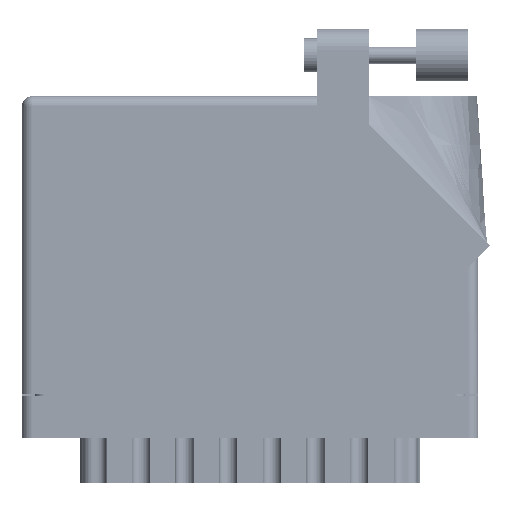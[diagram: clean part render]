
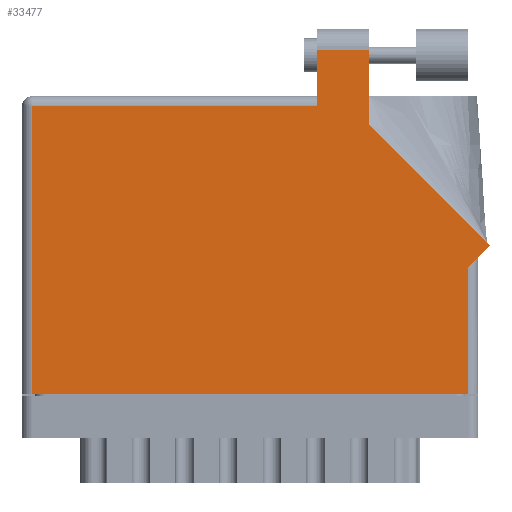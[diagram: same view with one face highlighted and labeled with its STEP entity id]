
A CAD part, front view. The second image highlights one B-rep face of the part: STEP entity #33477.
In plain terms, the highlighted face is planar.
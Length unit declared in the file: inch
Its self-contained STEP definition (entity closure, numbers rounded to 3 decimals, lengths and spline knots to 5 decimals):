
#1306 = DIRECTION ( 'NONE',  ( -1., 0., 0. ) ) ;
#2061 = DIRECTION ( 'NONE',  ( 0., 0., -1. ) ) ;
#2221 = VECTOR ( 'NONE', #69357, 39.37008 ) ;
#2940 = LINE ( 'NONE', #4079, #55872 ) ;
#4079 = CARTESIAN_POINT ( 'NONE',  ( 1.758, 2.05, 0. ) ) ;
#4353 = LINE ( 'NONE', #40347, #47713 ) ;
#5128 = ORIENTED_EDGE ( 'NONE', *, *, #47192, .T. ) ;
#6887 = CARTESIAN_POINT ( 'NONE',  ( 2.78871, 0.88571, 0. ) ) ;
#7478 = CARTESIAN_POINT ( 'NONE',  ( 0., 1.775, 0. ) ) ;
#8023 = DIRECTION ( 'NONE',  ( -0.707, 0.707, 0. ) ) ;
#9760 = CARTESIAN_POINT ( 'NONE',  ( 2.065, 1.60942, 0. ) ) ;
#12883 = EDGE_CURVE ( 'NONE', #18476, #69087, #34886, .T. ) ;
#13720 = LINE ( 'NONE', #59563, #61947 ) ;
#16546 = CARTESIAN_POINT ( 'NONE',  ( 2.78871, 0.88571, 0. ) ) ;
#18476 = VERTEX_POINT ( 'NONE', #27235 ) ;
#19517 = ORIENTED_EDGE ( 'NONE', *, *, #45539, .T. ) ;
#20413 = CARTESIAN_POINT ( 'NONE',  ( 2.065, 1.60942, 0. ) ) ;
#23013 = CARTESIAN_POINT ( 'NONE',  ( 0.062, 1.713, 0. ) ) ;
#24064 = ORIENTED_EDGE ( 'NONE', *, *, #57484, .T. ) ;
#24742 = CARTESIAN_POINT ( 'NONE',  ( 1.758, 1.775, 0. ) ) ;
#25111 = DIRECTION ( 'NONE',  ( 0., -1., 0. ) ) ;
#25293 = PLANE ( 'NONE',  #62700 ) ;
#25743 = EDGE_CURVE ( 'NONE', #68118, #18476, #13720, .T. ) ;
#25893 = DIRECTION ( 'NONE',  ( 0., -1., 0. ) ) ;
#27235 = CARTESIAN_POINT ( 'NONE',  ( 2.656, 0., 0. ) ) ;
#28054 = DIRECTION ( 'NONE',  ( -1., 0., 0. ) ) ;
#30588 = EDGE_CURVE ( 'NONE', #34172, #41704, #43676, .T. ) ;
#31691 = LINE ( 'NONE', #44059, #65145 ) ;
#33477 = ADVANCED_FACE ( 'NONE', ( #43479 ), #25293, .F. ) ;
#34172 = VERTEX_POINT ( 'NONE', #76593 ) ;
#34886 = LINE ( 'NONE', #51167, #2221 ) ;
#35531 = ORIENTED_EDGE ( 'NONE', *, *, #30588, .T. ) ;
#35906 = VERTEX_POINT ( 'NONE', #16546 ) ;
#39192 = ORIENTED_EDGE ( 'NONE', *, *, #41497, .T. ) ;
#40347 = CARTESIAN_POINT ( 'NONE',  ( 2.718, 0.815, 0. ) ) ;
#41497 = EDGE_CURVE ( 'NONE', #69766, #34172, #2940, .T. ) ;
#41634 = CARTESIAN_POINT ( 'NONE',  ( 0.062, 0., 0. ) ) ;
#41704 = VERTEX_POINT ( 'NONE', #54655 ) ;
#42881 = LINE ( 'NONE', #6887, #74792 ) ;
#42973 = CARTESIAN_POINT ( 'NONE',  ( 2.656, 0.753, 0. ) ) ;
#43479 = FACE_OUTER_BOUND ( 'NONE', #75361, .T. ) ;
#43676 = LINE ( 'NONE', #24742, #59876 ) ;
#44059 = CARTESIAN_POINT ( 'NONE',  ( 0.062, 0., 0. ) ) ;
#44790 = ORIENTED_EDGE ( 'NONE', *, *, #72641, .T. ) ;
#44981 = DIRECTION ( 'NONE',  ( 0., 1., 0. ) ) ;
#45090 = CARTESIAN_POINT ( 'NONE',  ( 0., 1.713, 0. ) ) ;
#45539 = EDGE_CURVE ( 'NONE', #41704, #61387, #75702, .T. ) ;
#47192 = EDGE_CURVE ( 'NONE', #69087, #35906, #4353, .T. ) ;
#47532 = DIRECTION ( 'NONE',  ( 1., 0., 0. ) ) ;
#47713 = VECTOR ( 'NONE', #62856, 39.37008 ) ;
#50979 = ORIENTED_EDGE ( 'NONE', *, *, #25743, .T. ) ;
#51167 = CARTESIAN_POINT ( 'NONE',  ( 2.656, 0.815, 0. ) ) ;
#52903 = VECTOR ( 'NONE', #44981, 39.37008 ) ;
#53953 = CARTESIAN_POINT ( 'NONE',  ( 2.065, 2.05, 0. ) ) ;
#54346 = EDGE_CURVE ( 'NONE', #61387, #68118, #31691, .T. ) ;
#54655 = CARTESIAN_POINT ( 'NONE',  ( 1.758, 1.713, 0. ) ) ;
#55872 = VECTOR ( 'NONE', #73834, 39.37008 ) ;
#57408 = VECTOR ( 'NONE', #28054, 39.37008 ) ;
#57484 = EDGE_CURVE ( 'NONE', #60877, #69766, #67487, .T. ) ;
#58801 = ORIENTED_EDGE ( 'NONE', *, *, #54346, .T. ) ;
#59563 = CARTESIAN_POINT ( 'NONE',  ( 0., 0., 0. ) ) ;
#59876 = VECTOR ( 'NONE', #25111, 39.37008 ) ;
#60877 = VERTEX_POINT ( 'NONE', #20413 ) ;
#61387 = VERTEX_POINT ( 'NONE', #23013 ) ;
#61947 = VECTOR ( 'NONE', #47532, 39.37008 ) ;
#62700 = AXIS2_PLACEMENT_3D ( 'NONE', #7478, #2061, #1306 ) ;
#62856 = DIRECTION ( 'NONE',  ( 0.707, 0.707, 0. ) ) ;
#63531 = ORIENTED_EDGE ( 'NONE', *, *, #12883, .T. ) ;
#65145 = VECTOR ( 'NONE', #25893, 39.37008 ) ;
#67487 = LINE ( 'NONE', #9760, #52903 ) ;
#68118 = VERTEX_POINT ( 'NONE', #41634 ) ;
#69087 = VERTEX_POINT ( 'NONE', #42973 ) ;
#69357 = DIRECTION ( 'NONE',  ( 0., 1., 0. ) ) ;
#69766 = VERTEX_POINT ( 'NONE', #53953 ) ;
#72641 = EDGE_CURVE ( 'NONE', #35906, #60877, #42881, .T. ) ;
#73834 = DIRECTION ( 'NONE',  ( -1., 0., 0. ) ) ;
#74792 = VECTOR ( 'NONE', #8023, 39.37008 ) ;
#75361 = EDGE_LOOP ( 'NONE', ( #24064, #39192, #35531, #19517, #58801, #50979, #63531, #5128, #44790 ) ) ;
#75702 = LINE ( 'NONE', #45090, #57408 ) ;
#76593 = CARTESIAN_POINT ( 'NONE',  ( 1.758, 2.05, 0. ) ) ;
